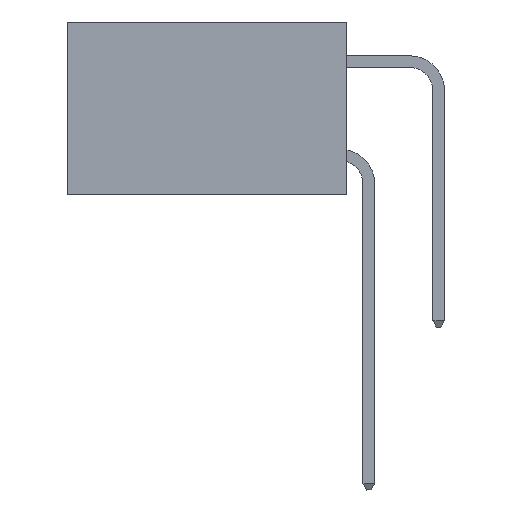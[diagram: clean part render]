
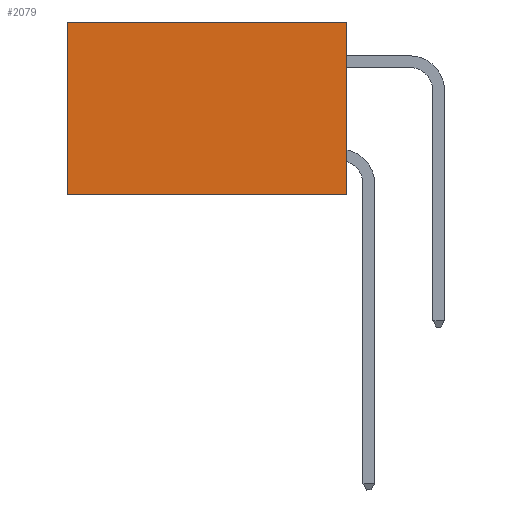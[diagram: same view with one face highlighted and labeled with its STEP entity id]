
A CAD part, left-side view. The second image highlights one B-rep face of the part: STEP entity #2079.
In plain terms, the highlighted planar face has unit normal (-1, 0, 0).
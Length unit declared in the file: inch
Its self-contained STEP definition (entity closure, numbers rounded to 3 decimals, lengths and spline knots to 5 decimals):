
#702 = LINE ( 'NONE', #2119, #8906 ) ;
#835 = AXIS2_PLACEMENT_3D ( 'NONE', #9877, #8828, #2184 ) ;
#1345 = CARTESIAN_POINT ( 'NONE',  ( 0.2875, 0., 0. ) ) ;
#1460 = DIRECTION ( 'NONE',  ( 0., 1., 0. ) ) ;
#1772 = LINE ( 'NONE', #6041, #9850 ) ;
#2079 = ADVANCED_FACE ( 'NONE', ( #2998 ), #7442, .F. ) ;
#2119 = CARTESIAN_POINT ( 'NONE',  ( 0.2875, 0., -0.37 ) ) ;
#2184 = DIRECTION ( 'NONE',  ( 0., 0., -1. ) ) ;
#2455 = ORIENTED_EDGE ( 'NONE', *, *, #5732, .T. ) ;
#2495 = CARTESIAN_POINT ( 'NONE',  ( 0.2875, 0.6, -0.37 ) ) ;
#2576 = VECTOR ( 'NONE', #3874, 39.37008 ) ;
#2836 = VERTEX_POINT ( 'NONE', #9900 ) ;
#2998 = FACE_OUTER_BOUND ( 'NONE', #5905, .T. ) ;
#3701 = VERTEX_POINT ( 'NONE', #2495 ) ;
#3874 = DIRECTION ( 'NONE',  ( 0., 0., -1. ) ) ;
#4079 = CARTESIAN_POINT ( 'NONE',  ( 0.2875, 0., -0.37 ) ) ;
#4180 = EDGE_CURVE ( 'NONE', #5254, #8633, #4985, .T. ) ;
#4692 = CARTESIAN_POINT ( 'NONE',  ( 0.2875, 0., 0. ) ) ;
#4874 = ORIENTED_EDGE ( 'NONE', *, *, #8491, .T. ) ;
#4985 = LINE ( 'NONE', #1345, #2576 ) ;
#5254 = VERTEX_POINT ( 'NONE', #4692 ) ;
#5373 = EDGE_CURVE ( 'NONE', #8633, #3701, #702, .T. ) ;
#5732 = EDGE_CURVE ( 'NONE', #2836, #3701, #1772, .T. ) ;
#5905 = EDGE_LOOP ( 'NONE', ( #2455, #6635, #9657, #4874 ) ) ;
#6041 = CARTESIAN_POINT ( 'NONE',  ( 0.2875, 0.6, 0. ) ) ;
#6635 = ORIENTED_EDGE ( 'NONE', *, *, #5373, .F. ) ;
#7442 = PLANE ( 'NONE',  #835 ) ;
#7775 = CARTESIAN_POINT ( 'NONE',  ( 0.2875, 0., 0. ) ) ;
#8309 = DIRECTION ( 'NONE',  ( 0., 0., -1. ) ) ;
#8491 = EDGE_CURVE ( 'NONE', #5254, #2836, #8973, .T. ) ;
#8633 = VERTEX_POINT ( 'NONE', #4079 ) ;
#8724 = DIRECTION ( 'NONE',  ( 0., 1., 0. ) ) ;
#8733 = VECTOR ( 'NONE', #1460, 39.37008 ) ;
#8828 = DIRECTION ( 'NONE',  ( 1., 0., 0. ) ) ;
#8906 = VECTOR ( 'NONE', #8724, 39.37008 ) ;
#8973 = LINE ( 'NONE', #7775, #8733 ) ;
#9657 = ORIENTED_EDGE ( 'NONE', *, *, #4180, .F. ) ;
#9850 = VECTOR ( 'NONE', #8309, 39.37008 ) ;
#9877 = CARTESIAN_POINT ( 'NONE',  ( 0.2875, 0., 0. ) ) ;
#9900 = CARTESIAN_POINT ( 'NONE',  ( 0.2875, 0.6, 0. ) ) ;
